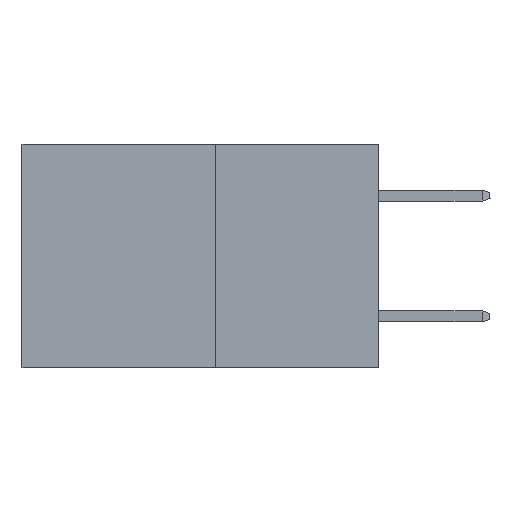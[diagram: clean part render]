
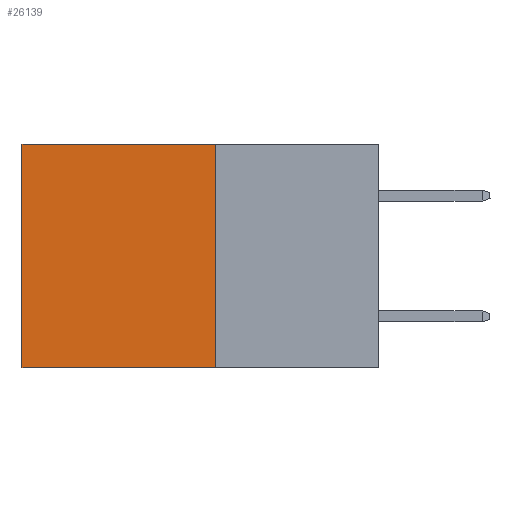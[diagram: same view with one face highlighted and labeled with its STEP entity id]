
A CAD part, left-side view. The second image highlights one B-rep face of the part: STEP entity #26139.
In plain terms, the highlighted planar face has unit normal (-1, 0, 0).
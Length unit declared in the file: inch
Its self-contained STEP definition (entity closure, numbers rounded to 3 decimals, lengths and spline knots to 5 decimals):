
#604 = VERTEX_POINT ( 'NONE', #2922 ) ;
#1221 = LINE ( 'NONE', #6019, #18413 ) ;
#1346 = ORIENTED_EDGE ( 'NONE', *, *, #4032, .F. ) ;
#1572 = DIRECTION ( 'NONE',  ( 0., 0., -1. ) ) ;
#2658 = EDGE_CURVE ( 'NONE', #11399, #30218, #27162, .T. ) ;
#2922 = CARTESIAN_POINT ( 'NONE',  ( 0.277, 0.59, -0.37 ) ) ;
#3765 = LINE ( 'NONE', #25273, #15413 ) ;
#4032 = EDGE_CURVE ( 'NONE', #30218, #604, #3765, .T. ) ;
#4719 = FACE_OUTER_BOUND ( 'NONE', #11392, .T. ) ;
#6019 = CARTESIAN_POINT ( 'NONE',  ( 0.277, 0.59, -0.37 ) ) ;
#6461 = ORIENTED_EDGE ( 'NONE', *, *, #13546, .T. ) ;
#7924 = ORIENTED_EDGE ( 'NONE', *, *, #2658, .F. ) ;
#8396 = VECTOR ( 'NONE', #19281, 39.37008 ) ;
#8775 = DIRECTION ( 'NONE',  ( 0., 0., -1. ) ) ;
#9285 = AXIS2_PLACEMENT_3D ( 'NONE', #29501, #15596, #1572 ) ;
#10710 = DIRECTION ( 'NONE',  ( 0., 0., -1. ) ) ;
#11392 = EDGE_LOOP ( 'NONE', ( #22158, #1346, #7924, #6461 ) ) ;
#11399 = VERTEX_POINT ( 'NONE', #18878 ) ;
#13267 = PLANE ( 'NONE',  #9285 ) ;
#13546 = EDGE_CURVE ( 'NONE', #11399, #27808, #20786, .T. ) ;
#15413 = VECTOR ( 'NONE', #18335, 39.37008 ) ;
#15596 = DIRECTION ( 'NONE',  ( 1., 0., 0. ) ) ;
#16965 = CARTESIAN_POINT ( 'NONE',  ( 0.277, 0.27, 0. ) ) ;
#17449 = CARTESIAN_POINT ( 'NONE',  ( 0.277, 0.27, -0.37 ) ) ;
#17997 = CARTESIAN_POINT ( 'NONE',  ( 0.277, 0.27, -0.37 ) ) ;
#18335 = DIRECTION ( 'NONE',  ( 0., 1., 0. ) ) ;
#18413 = VECTOR ( 'NONE', #10710, 39.37008 ) ;
#18878 = CARTESIAN_POINT ( 'NONE',  ( 0.277, 0.27, 0. ) ) ;
#19281 = DIRECTION ( 'NONE',  ( 0., 1., 0. ) ) ;
#20786 = LINE ( 'NONE', #16965, #8396 ) ;
#20957 = CARTESIAN_POINT ( 'NONE',  ( 0.277, 0.59, 0. ) ) ;
#20986 = VECTOR ( 'NONE', #8775, 39.37008 ) ;
#22158 = ORIENTED_EDGE ( 'NONE', *, *, #22254, .T. ) ;
#22254 = EDGE_CURVE ( 'NONE', #27808, #604, #1221, .T. ) ;
#25273 = CARTESIAN_POINT ( 'NONE',  ( 0.277, 0.27, -0.37 ) ) ;
#26139 = ADVANCED_FACE ( 'NONE', ( #4719 ), #13267, .F. ) ;
#27162 = LINE ( 'NONE', #17997, #20986 ) ;
#27808 = VERTEX_POINT ( 'NONE', #20957 ) ;
#29501 = CARTESIAN_POINT ( 'NONE',  ( 0.277, 0.27, -0.37 ) ) ;
#30218 = VERTEX_POINT ( 'NONE', #17449 ) ;
